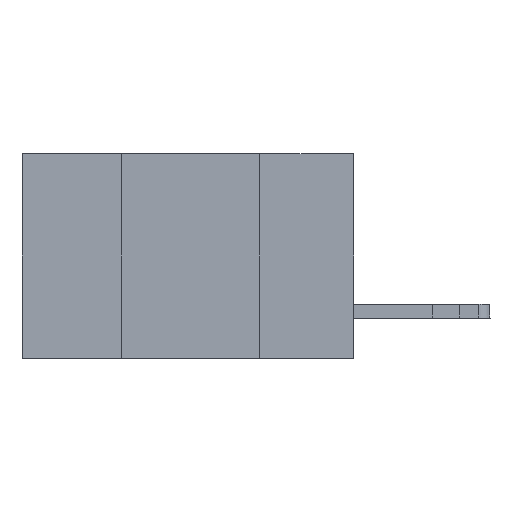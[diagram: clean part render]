
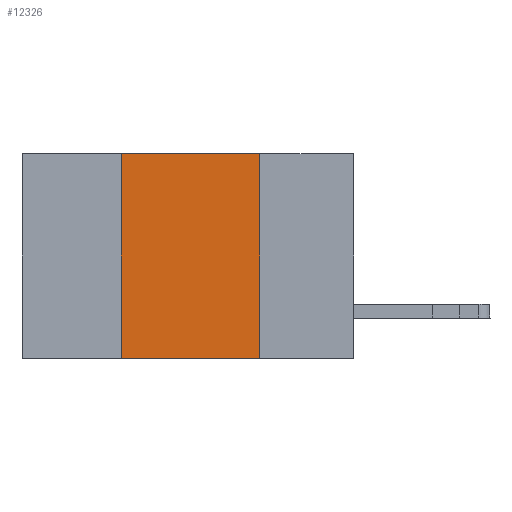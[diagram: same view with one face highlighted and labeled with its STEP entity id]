
A CAD part, left-side view. The second image highlights one B-rep face of the part: STEP entity #12326.
In plain terms, the highlighted planar face has unit normal (-1, 0, 0).
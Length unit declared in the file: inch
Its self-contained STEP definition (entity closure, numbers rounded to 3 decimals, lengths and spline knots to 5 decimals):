
#297 = EDGE_CURVE ( 'NONE', #12091, #15339, #20811, .T. ) ;
#1484 = ORIENTED_EDGE ( 'NONE', *, *, #4216, .T. ) ;
#1722 = ORIENTED_EDGE ( 'NONE', *, *, #17179, .F. ) ;
#3047 = VECTOR ( 'NONE', #14264, 39.37008 ) ;
#3671 = EDGE_CURVE ( 'NONE', #15339, #20685, #17124, .T. ) ;
#4216 = EDGE_CURVE ( 'NONE', #12091, #22338, #11903, .T. ) ;
#6187 = ORIENTED_EDGE ( 'NONE', *, *, #3671, .F. ) ;
#7195 = DIRECTION ( 'NONE',  ( 0., -1., 0. ) ) ;
#7742 = VECTOR ( 'NONE', #7195, 39.37008 ) ;
#10104 = CARTESIAN_POINT ( 'NONE',  ( 0., 0.6, 0. ) ) ;
#11359 = AXIS2_PLACEMENT_3D ( 'NONE', #10104, #22354, #11860 ) ;
#11860 = DIRECTION ( 'NONE',  ( 0., 0., -1. ) ) ;
#11903 = LINE ( 'NONE', #17433, #20664 ) ;
#12051 = FACE_OUTER_BOUND ( 'NONE', #17317, .T. ) ;
#12091 = VERTEX_POINT ( 'NONE', #16470 ) ;
#12326 = ADVANCED_FACE ( 'NONE', ( #12051 ), #20586, .F. ) ;
#12498 = CARTESIAN_POINT ( 'NONE',  ( 0., 0.17, 0. ) ) ;
#14234 = CARTESIAN_POINT ( 'NONE',  ( 0., 0.6, 0. ) ) ;
#14264 = DIRECTION ( 'NONE',  ( 0., 0., -1. ) ) ;
#15339 = VERTEX_POINT ( 'NONE', #19393 ) ;
#16156 = VECTOR ( 'NONE', #19392, 39.37008 ) ;
#16470 = CARTESIAN_POINT ( 'NONE',  ( 0., 0.42, -0.37 ) ) ;
#17124 = LINE ( 'NONE', #14234, #7742 ) ;
#17179 = EDGE_CURVE ( 'NONE', #20685, #22338, #21875, .T. ) ;
#17317 = EDGE_LOOP ( 'NONE', ( #1722, #6187, #21187, #1484 ) ) ;
#17433 = CARTESIAN_POINT ( 'NONE',  ( 0., 0.6, -0.37 ) ) ;
#18137 = CARTESIAN_POINT ( 'NONE',  ( 0., 0.17, 0. ) ) ;
#19201 = DIRECTION ( 'NONE',  ( 0., -1., 0. ) ) ;
#19392 = DIRECTION ( 'NONE',  ( 0., 0., 1. ) ) ;
#19393 = CARTESIAN_POINT ( 'NONE',  ( 0., 0.42, 0. ) ) ;
#20586 = PLANE ( 'NONE',  #11359 ) ;
#20664 = VECTOR ( 'NONE', #19201, 39.37008 ) ;
#20685 = VERTEX_POINT ( 'NONE', #18137 ) ;
#20811 = LINE ( 'NONE', #20917, #16156 ) ;
#20917 = CARTESIAN_POINT ( 'NONE',  ( 0., 0.42, 0. ) ) ;
#21187 = ORIENTED_EDGE ( 'NONE', *, *, #297, .F. ) ;
#21875 = LINE ( 'NONE', #12498, #3047 ) ;
#22338 = VERTEX_POINT ( 'NONE', #22654 ) ;
#22354 = DIRECTION ( 'NONE',  ( 1., 0., 0. ) ) ;
#22654 = CARTESIAN_POINT ( 'NONE',  ( 0., 0.17, -0.37 ) ) ;
